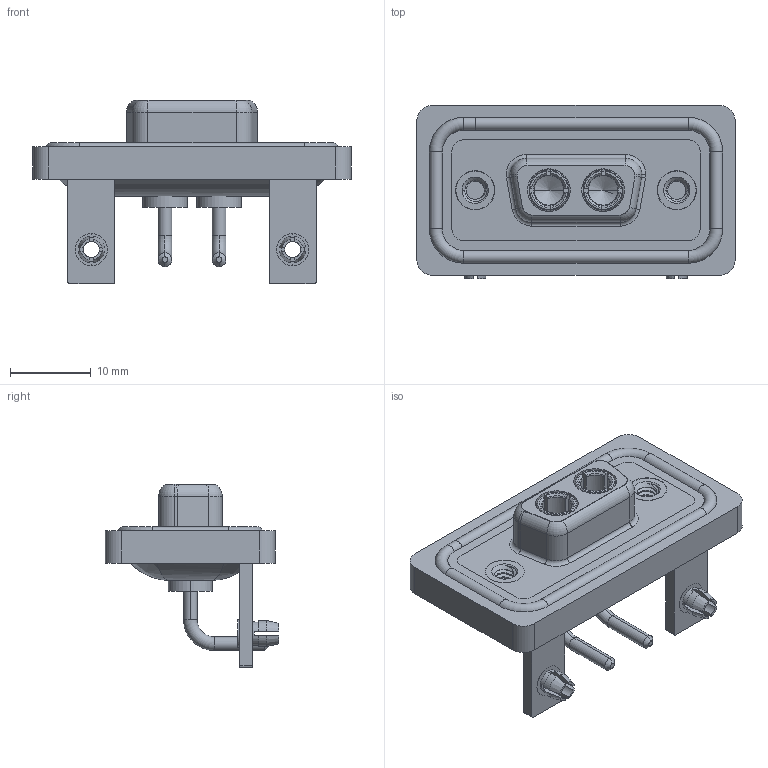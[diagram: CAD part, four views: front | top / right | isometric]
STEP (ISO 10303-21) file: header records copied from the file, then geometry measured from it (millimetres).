
FILE_DESCRIPTION (( 'STEP AP203' ), '1' );
FILE_NAME ('630W2W2-640-1N3.STEP', '2024-04-11T21:05:14', ( '' ), ( '' ), 'SwSTEP 2.0', 'SolidWorks 2023', '' );
FILE_SCHEMA (( 'CONFIG_CONTROL_DESIGN' ));
Length unit declared in the file: millimetre
Products named in the file (9): 630Combo Threaded Rivet_2; 630Combo Waterproof Housing_09 Contacts; 630W2W2-640-1N3; 630Combo Housing_2W2; 630Combo Board Lock_50 Contacts; Power Socket_10A RA; 630Combo Shell Rear_09 Contacts; 630Combo Stabilizer Bracket_50 Contacts; 630Combo Shell Front_09 Contacts
Assembly tree (12 placements, depth 2):
  630W2W2-640-1N3
    630Combo Housing_2W2
    630Combo Shell Front_09 Contacts
    630Combo Shell Rear_09 Contacts
    630Combo Threaded Rivet_2  x2
    630Combo Stabilizer Bracket_50 Contacts  x2
    630Combo Board Lock_50 Contacts  x2
    Power Socket_10A RA  x2
    630Combo Waterproof Housing_09 Contacts
Bounding box: 39.5 x 21.5 x 22.8 mm (x, y, z)
Volume: 5103.2 mm3; surface area: 8630.2 mm2
Topology: 15 solids, 15 shells, 682 faces, 1733 edges, 1100 vertices
Faces by surface type: cylinder 294, plane 231, torus 83, cone 62, bspline 12
Entity records: 18220 total; most frequent: CARTESIAN_POINT 4858, DIRECTION 2708, ORIENTED_EDGE 2528, EDGE_CURVE 1264, AXIS2_PLACEMENT_3D 1072, VERTEX_POINT 801, LINE 564, VECTOR 564
